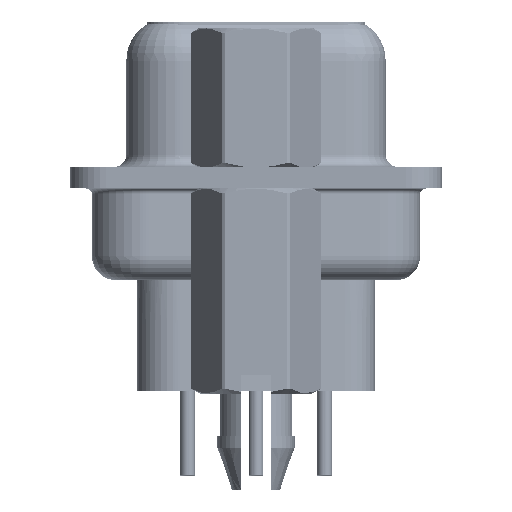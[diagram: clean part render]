
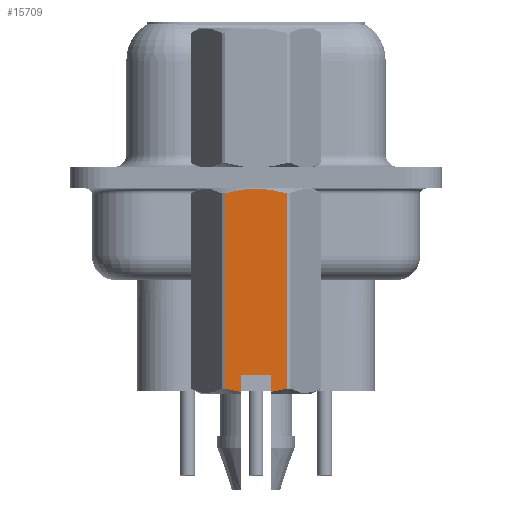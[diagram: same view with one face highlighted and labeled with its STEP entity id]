
A CAD part, left-side view. The second image highlights one B-rep face of the part: STEP entity #15709.
In plain terms, the highlighted planar face has unit normal (-1, 0, 0).
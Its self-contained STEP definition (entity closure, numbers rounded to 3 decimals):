
#2078 = EDGE_CURVE ( 'NONE', #62513, #59185, #38040, .T. ) ;
#2090 = CARTESIAN_POINT ( 'NONE',  ( -2.381, 0.625, -8.2 ) ) ;
#4154 = CARTESIAN_POINT ( 'NONE',  ( -2.381, -0.215, -0.468 ) ) ;
#4530 = DIRECTION ( 'NONE',  ( -1., 0., 0. ) ) ;
#6273 = EDGE_LOOP ( 'NONE', ( #31500, #20267, #56110, #61390, #42348, #62392, #36849, #24169, #32745 ) ) ;
#7525 = EDGE_CURVE ( 'NONE', #67262, #41374, #18920, .T. ) ;
#8661 = CARTESIAN_POINT ( 'NONE',  ( -2.381, -1.273, -0.652 ) ) ;
#9652 = DIRECTION ( 'NONE',  ( 0., 0., 1. ) ) ;
#11498 = LINE ( 'NONE', #21764, #42222 ) ;
#12057 = DIRECTION ( 'NONE',  ( 0., 0., -1. ) ) ;
#14738 = CARTESIAN_POINT ( 'NONE',  ( -2.381, -1.065, -0.596 ) ) ;
#15709 = ADVANCED_FACE ( 'NONE', ( #26376 ), #62928, .T. ) ;
#16279 = CARTESIAN_POINT ( 'NONE',  ( -2.381, 1.06, -8.806 ) ) ;
#17530 = VECTOR ( 'NONE', #20057, 1000. ) ;
#18920 = B_SPLINE_CURVE_WITH_KNOTS ( 'NONE', 3,
 ( #31259, #52099, #53462, #52775, #37395, #36379 ),
 .UNSPECIFIED., .F., .F.,
 ( 4, 2, 4 ),
 ( 0.004, 0.004, 0.005 ),
 .UNSPECIFIED. ) ;
#19190 = CARTESIAN_POINT ( 'NONE',  ( -2.381, 0., -0.468 ) ) ;
#20057 = DIRECTION ( 'NONE',  ( 0., 0., -1. ) ) ;
#20233 = CARTESIAN_POINT ( 'NONE',  ( -2.381, -1.375, 7.399 ) ) ;
#20267 = ORIENTED_EDGE ( 'NONE', *, *, #22748, .F. ) ;
#21250 = CARTESIAN_POINT ( 'NONE',  ( -2.381, -1.06, -8.806 ) ) ;
#21764 = CARTESIAN_POINT ( 'NONE',  ( -2.381, 1.273, 0.581 ) ) ;
#22508 = CARTESIAN_POINT ( 'NONE',  ( -2.381, -0.625, -8.885 ) ) ;
#22615 = EDGE_CURVE ( 'NONE', #59630, #46021, #25553, .T. ) ;
#22748 = EDGE_CURVE ( 'NONE', #62513, #67092, #42312, .T. ) ;
#22774 = CARTESIAN_POINT ( 'NONE',  ( -2.381, 1.273, -8.748 ) ) ;
#24169 = ORIENTED_EDGE ( 'NONE', *, *, #34744, .T. ) ;
#24307 = CARTESIAN_POINT ( 'NONE',  ( -2.381, -1.273, -0.652 ) ) ;
#24312 = VERTEX_POINT ( 'NONE', #57330 ) ;
#25496 = CARTESIAN_POINT ( 'NONE',  ( -2.381, 0.625, -8.885 ) ) ;
#25510 = CARTESIAN_POINT ( 'NONE',  ( -2.381, 0.625, -8.2 ) ) ;
#25553 = LINE ( 'NONE', #35155, #38711 ) ;
#26376 = FACE_OUTER_BOUND ( 'NONE', #6273, .T. ) ;
#27029 = B_SPLINE_CURVE_WITH_KNOTS ( 'NONE', 3,
 ( #24307, #14738, #29785, #30482, #4154, #19190 ),
 .UNSPECIFIED., .F., .F.,
 ( 4, 2, 4 ),
 ( 0.003, 0.003, 0.004 ),
 .UNSPECIFIED. ) ;
#27961 = EDGE_CURVE ( 'NONE', #30228, #24312, #30587, .T. ) ;
#29785 = CARTESIAN_POINT ( 'NONE',  ( -2.381, -0.853, -0.549 ) ) ;
#30228 = VERTEX_POINT ( 'NONE', #22774 ) ;
#30482 = CARTESIAN_POINT ( 'NONE',  ( -2.381, -0.428, -0.485 ) ) ;
#30587 = B_SPLINE_CURVE_WITH_KNOTS ( 'NONE', 3,
 ( #35770, #16279, #47374, #25496 ),
 .UNSPECIFIED., .F., .F.,
 ( 4, 4 ),
 ( 0.001, 0.002 ),
 .UNSPECIFIED. ) ;
#31259 = CARTESIAN_POINT ( 'NONE',  ( -2.381, 0., -0.468 ) ) ;
#31375 = CARTESIAN_POINT ( 'NONE',  ( -2.381, -0.625, -8.2 ) ) ;
#31500 = ORIENTED_EDGE ( 'NONE', *, *, #48847, .F. ) ;
#32745 = ORIENTED_EDGE ( 'NONE', *, *, #27961, .T. ) ;
#34744 = EDGE_CURVE ( 'NONE', #41374, #30228, #11498, .T. ) ;
#35002 = B_SPLINE_CURVE_WITH_KNOTS ( 'NONE', 3,
 ( #47229, #47566, #21250, #52355 ),
 .UNSPECIFIED., .F., .F.,
 ( 4, 4 ),
 ( 0.003, 0.004 ),
 .UNSPECIFIED. ) ;
#35155 = CARTESIAN_POINT ( 'NONE',  ( -2.381, -1.273, 0.581 ) ) ;
#35770 = CARTESIAN_POINT ( 'NONE',  ( -2.381, 1.273, -8.748 ) ) ;
#36170 = DIRECTION ( 'NONE',  ( 0., 0., 1. ) ) ;
#36379 = CARTESIAN_POINT ( 'NONE',  ( -2.381, 1.273, -0.652 ) ) ;
#36849 = ORIENTED_EDGE ( 'NONE', *, *, #7525, .T. ) ;
#37395 = CARTESIAN_POINT ( 'NONE',  ( -2.381, 1.066, -0.596 ) ) ;
#38040 = LINE ( 'NONE', #58865, #59664 ) ;
#38176 = AXIS2_PLACEMENT_3D ( 'NONE', #20233, #4530, #9652 ) ;
#38711 = VECTOR ( 'NONE', #36170, 1000. ) ;
#41374 = VERTEX_POINT ( 'NONE', #56913 ) ;
#42222 = VECTOR ( 'NONE', #43624, 1000. ) ;
#42312 = LINE ( 'NONE', #31375, #60519 ) ;
#42348 = ORIENTED_EDGE ( 'NONE', *, *, #22615, .T. ) ;
#43624 = DIRECTION ( 'NONE',  ( 0., 0., -1. ) ) ;
#46021 = VERTEX_POINT ( 'NONE', #8661 ) ;
#46714 = LINE ( 'NONE', #25510, #17530 ) ;
#47229 = CARTESIAN_POINT ( 'NONE',  ( -2.381, -0.625, -8.885 ) ) ;
#47374 = CARTESIAN_POINT ( 'NONE',  ( -2.381, 0.845, -8.853 ) ) ;
#47392 = CARTESIAN_POINT ( 'NONE',  ( -2.381, -1.273, -8.748 ) ) ;
#47566 = CARTESIAN_POINT ( 'NONE',  ( -2.381, -0.842, -8.854 ) ) ;
#48847 = EDGE_CURVE ( 'NONE', #67092, #24312, #46714, .T. ) ;
#49508 = CARTESIAN_POINT ( 'NONE',  ( -2.381, -0.625, -8.2 ) ) ;
#52099 = CARTESIAN_POINT ( 'NONE',  ( -2.381, 0.215, -0.468 ) ) ;
#52355 = CARTESIAN_POINT ( 'NONE',  ( -2.381, -1.273, -8.748 ) ) ;
#52775 = CARTESIAN_POINT ( 'NONE',  ( -2.381, 0.858, -0.55 ) ) ;
#53462 = CARTESIAN_POINT ( 'NONE',  ( -2.381, 0.432, -0.485 ) ) ;
#56110 = ORIENTED_EDGE ( 'NONE', *, *, #2078, .T. ) ;
#56913 = CARTESIAN_POINT ( 'NONE',  ( -2.381, 1.273, -0.652 ) ) ;
#57330 = CARTESIAN_POINT ( 'NONE',  ( -2.381, 0.625, -8.885 ) ) ;
#57501 = EDGE_CURVE ( 'NONE', #46021, #67262, #27029, .T. ) ;
#58865 = CARTESIAN_POINT ( 'NONE',  ( -2.381, -0.625, -8.2 ) ) ;
#59185 = VERTEX_POINT ( 'NONE', #22508 ) ;
#59630 = VERTEX_POINT ( 'NONE', #47392 ) ;
#59664 = VECTOR ( 'NONE', #12057, 1000. ) ;
#60124 = CARTESIAN_POINT ( 'NONE',  ( -2.381, 0., -0.468 ) ) ;
#60519 = VECTOR ( 'NONE', #63801, 1000. ) ;
#60570 = EDGE_CURVE ( 'NONE', #59185, #59630, #35002, .T. ) ;
#61390 = ORIENTED_EDGE ( 'NONE', *, *, #60570, .T. ) ;
#62392 = ORIENTED_EDGE ( 'NONE', *, *, #57501, .T. ) ;
#62513 = VERTEX_POINT ( 'NONE', #49508 ) ;
#62928 = PLANE ( 'NONE',  #38176 ) ;
#63801 = DIRECTION ( 'NONE',  ( 0., 1., 0. ) ) ;
#67092 = VERTEX_POINT ( 'NONE', #2090 ) ;
#67262 = VERTEX_POINT ( 'NONE', #60124 ) ;
